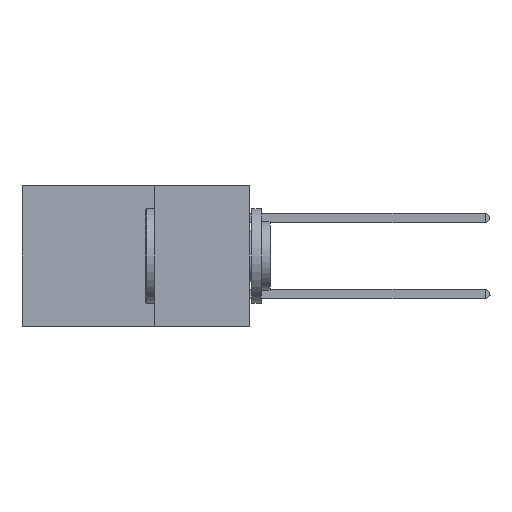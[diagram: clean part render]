
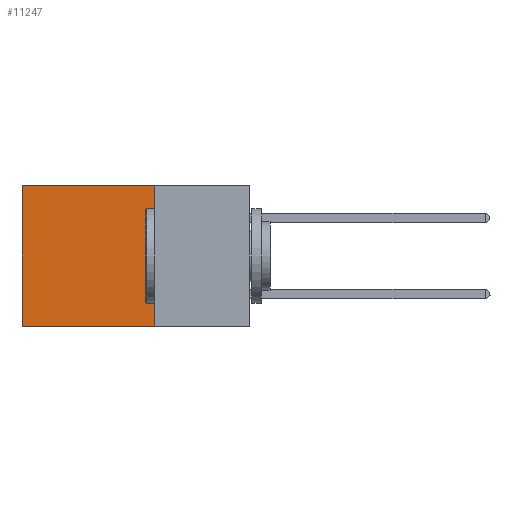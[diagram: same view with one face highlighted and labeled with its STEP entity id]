
A CAD part, left-side view. The second image highlights one B-rep face of the part: STEP entity #11247.
In plain terms, the highlighted planar face has unit normal (-1, 0, 0).
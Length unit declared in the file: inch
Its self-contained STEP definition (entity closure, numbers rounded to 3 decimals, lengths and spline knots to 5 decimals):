
#63 = CARTESIAN_POINT ( 'NONE',  ( 0.2875, 0.6, 0. ) ) ;
#90 = EDGE_CURVE ( 'NONE', #5782, #3251, #873, .T. ) ;
#266 = CARTESIAN_POINT ( 'NONE',  ( 0.2875, 0.6, -0.37 ) ) ;
#458 = EDGE_CURVE ( 'NONE', #13248, #2303, #14056, .T. ) ;
#864 = DIRECTION ( 'NONE',  ( 1., 0., 0. ) ) ;
#873 = LINE ( 'NONE', #3512, #7555 ) ;
#918 = EDGE_LOOP ( 'NONE', ( #5984, #11075, #1575, #2002 ) ) ;
#1575 = ORIENTED_EDGE ( 'NONE', *, *, #7602, .F. ) ;
#1769 = VECTOR ( 'NONE', #6716, 39.37008 ) ;
#2002 = ORIENTED_EDGE ( 'NONE', *, *, #458, .T. ) ;
#2088 = EDGE_CURVE ( 'NONE', #2303, #3251, #11616, .T. ) ;
#2176 = CARTESIAN_POINT ( 'NONE',  ( 0.2875, 0.25, 0. ) ) ;
#2303 = VERTEX_POINT ( 'NONE', #63 ) ;
#2792 = FACE_OUTER_BOUND ( 'NONE', #918, .T. ) ;
#3251 = VERTEX_POINT ( 'NONE', #266 ) ;
#3512 = CARTESIAN_POINT ( 'NONE',  ( 0.2875, 0.25, -0.37 ) ) ;
#4855 = AXIS2_PLACEMENT_3D ( 'NONE', #8982, #864, #9028 ) ;
#5782 = VERTEX_POINT ( 'NONE', #12801 ) ;
#5984 = ORIENTED_EDGE ( 'NONE', *, *, #2088, .T. ) ;
#6716 = DIRECTION ( 'NONE',  ( 0., 0., -1. ) ) ;
#7162 = CARTESIAN_POINT ( 'NONE',  ( 0.2875, 0.25, 0. ) ) ;
#7555 = VECTOR ( 'NONE', #8574, 39.37008 ) ;
#7602 = EDGE_CURVE ( 'NONE', #13248, #5782, #10935, .T. ) ;
#7935 = PLANE ( 'NONE',  #4855 ) ;
#8574 = DIRECTION ( 'NONE',  ( 0., 1., 0. ) ) ;
#8982 = CARTESIAN_POINT ( 'NONE',  ( 0.2875, 0.25, 0. ) ) ;
#9028 = DIRECTION ( 'NONE',  ( 0., 0., -1. ) ) ;
#9230 = DIRECTION ( 'NONE',  ( 0., 0., -1. ) ) ;
#10935 = LINE ( 'NONE', #14399, #1769 ) ;
#11075 = ORIENTED_EDGE ( 'NONE', *, *, #90, .F. ) ;
#11247 = ADVANCED_FACE ( 'NONE', ( #2792 ), #7935, .F. ) ;
#11616 = LINE ( 'NONE', #12971, #14522 ) ;
#12801 = CARTESIAN_POINT ( 'NONE',  ( 0.2875, 0.25, -0.37 ) ) ;
#12971 = CARTESIAN_POINT ( 'NONE',  ( 0.2875, 0.6, 0. ) ) ;
#13248 = VERTEX_POINT ( 'NONE', #7162 ) ;
#13431 = DIRECTION ( 'NONE',  ( 0., 1., 0. ) ) ;
#14056 = LINE ( 'NONE', #2176, #14735 ) ;
#14399 = CARTESIAN_POINT ( 'NONE',  ( 0.2875, 0.25, 0. ) ) ;
#14522 = VECTOR ( 'NONE', #9230, 39.37008 ) ;
#14735 = VECTOR ( 'NONE', #13431, 39.37008 ) ;
